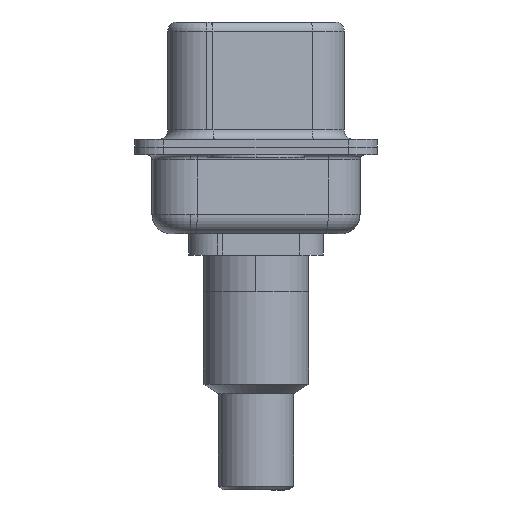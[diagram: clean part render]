
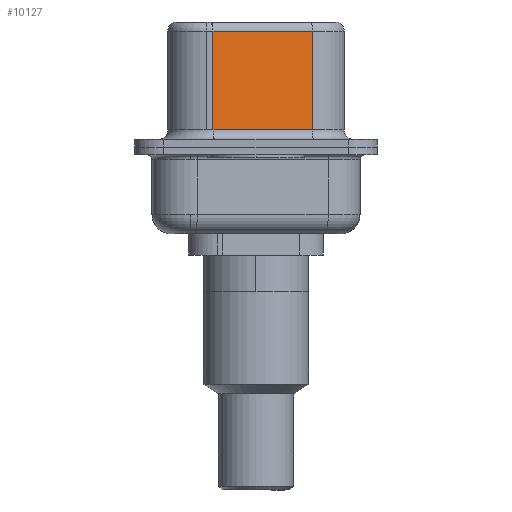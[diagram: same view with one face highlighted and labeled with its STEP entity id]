
A CAD part, left-side view. The second image highlights one B-rep face of the part: STEP entity #10127.
In plain terms, the highlighted planar face has unit normal (-0.985, -0.174, 0).
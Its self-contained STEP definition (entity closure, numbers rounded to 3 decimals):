
#658 = LINE ( 'NONE', #20513, #15013 ) ;
#2956 = CARTESIAN_POINT ( 'NONE',  ( 3.67, 2.233, 6.02 ) ) ;
#3217 = CARTESIAN_POINT ( 'NONE',  ( 4.58, -2.927, 0.9 ) ) ;
#3454 = CARTESIAN_POINT ( 'NONE',  ( 4.58, -2.927, 6.02 ) ) ;
#4715 = PLANE ( 'NONE',  #11860 ) ;
#4910 = ORIENTED_EDGE ( 'NONE', *, *, #15917, .F. ) ;
#5578 = EDGE_CURVE ( 'NONE', #23585, #21135, #16850, .T. ) ;
#6659 = DIRECTION ( 'NONE',  ( 0.985, 0.174, 0. ) ) ;
#8753 = VECTOR ( 'NONE', #14812, 1000. ) ;
#8892 = VERTEX_POINT ( 'NONE', #21648 ) ;
#8964 = VERTEX_POINT ( 'NONE', #3217 ) ;
#9361 = LINE ( 'NONE', #3454, #8753 ) ;
#9445 = DIRECTION ( 'NONE',  ( 0.174, -0.985, 0. ) ) ;
#9914 = CARTESIAN_POINT ( 'NONE',  ( 4.58, -2.927, 6.52 ) ) ;
#10127 = ADVANCED_FACE ( 'NONE', ( #20345 ), #4715, .F. ) ;
#10827 = LINE ( 'NONE', #9914, #14600 ) ;
#11860 = AXIS2_PLACEMENT_3D ( 'NONE', #19568, #6659, #19650 ) ;
#11938 = VECTOR ( 'NONE', #13041, 1000. ) ;
#12395 = EDGE_CURVE ( 'NONE', #21135, #8964, #658, .T. ) ;
#12734 = CARTESIAN_POINT ( 'NONE',  ( 3.67, 2.233, 6.52 ) ) ;
#13041 = DIRECTION ( 'NONE',  ( 0., 0., -1. ) ) ;
#14307 = ORIENTED_EDGE ( 'NONE', *, *, #12395, .T. ) ;
#14600 = VECTOR ( 'NONE', #22867, 1000. ) ;
#14812 = DIRECTION ( 'NONE',  ( -0.174, 0.985, 0. ) ) ;
#15013 = VECTOR ( 'NONE', #9445, 1000. ) ;
#15655 = EDGE_CURVE ( 'NONE', #8892, #23585, #9361, .T. ) ;
#15917 = EDGE_CURVE ( 'NONE', #8892, #8964, #10827, .T. ) ;
#16579 = CARTESIAN_POINT ( 'NONE',  ( 3.67, 2.233, 0.9 ) ) ;
#16850 = LINE ( 'NONE', #12734, #11938 ) ;
#18156 = ORIENTED_EDGE ( 'NONE', *, *, #5578, .T. ) ;
#19568 = CARTESIAN_POINT ( 'NONE',  ( 4.58, -2.927, 6.52 ) ) ;
#19650 = DIRECTION ( 'NONE',  ( -0.174, 0.985, 0. ) ) ;
#20345 = FACE_OUTER_BOUND ( 'NONE', #22772, .T. ) ;
#20382 = ORIENTED_EDGE ( 'NONE', *, *, #15655, .T. ) ;
#20513 = CARTESIAN_POINT ( 'NONE',  ( 4.58, -2.927, 0.9 ) ) ;
#21135 = VERTEX_POINT ( 'NONE', #16579 ) ;
#21648 = CARTESIAN_POINT ( 'NONE',  ( 4.58, -2.927, 6.02 ) ) ;
#22772 = EDGE_LOOP ( 'NONE', ( #4910, #20382, #18156, #14307 ) ) ;
#22867 = DIRECTION ( 'NONE',  ( 0., 0., -1. ) ) ;
#23585 = VERTEX_POINT ( 'NONE', #2956 ) ;
